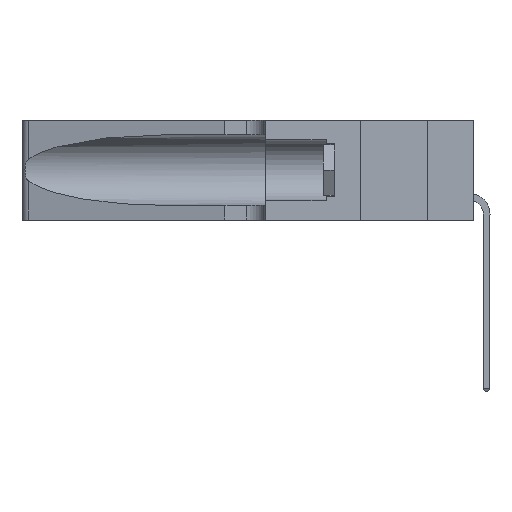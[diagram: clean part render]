
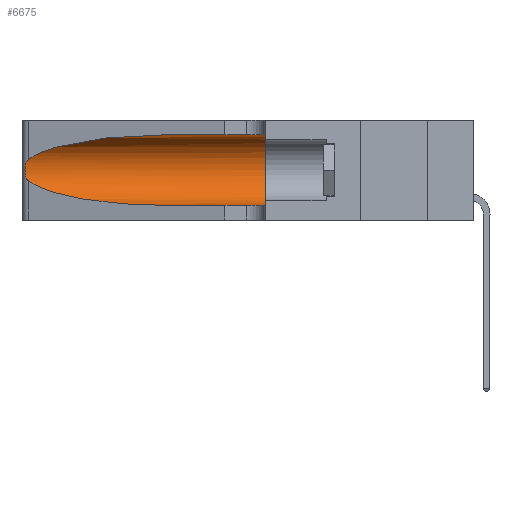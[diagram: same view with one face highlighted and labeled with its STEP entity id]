
A CAD part, left-side view. The second image highlights one B-rep face of the part: STEP entity #6675.
In plain terms, the highlighted cylindrical face has radius 3.308 mm (diameter 6.617 mm), a partial arc.
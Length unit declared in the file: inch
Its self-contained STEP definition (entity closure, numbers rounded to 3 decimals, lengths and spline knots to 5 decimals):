
#290 = LINE ( 'NONE', #19029, #35016 ) ;
#649 = CARTESIAN_POINT ( 'NONE',  ( 0.25639, 1.23186, 0.15144 ) ) ;
#1026 = AXIS2_PLACEMENT_3D ( 'NONE', #22013, #27946, #5043 ) ;
#2391 = ORIENTED_EDGE ( 'NONE', *, *, #7420, .T. ) ;
#3437 = VERTEX_POINT ( 'NONE', #31446 ) ;
#3533 = EDGE_LOOP ( 'NONE', ( #34411, #16324, #2391, #28532, #27664, #22790 ) ) ;
#3738 = CARTESIAN_POINT ( 'NONE',  ( 0.1305, 0.35, 0.185 ) ) ;
#4274 = FACE_OUTER_BOUND ( 'NONE', #3533, .T. ) ;
#4595 = CARTESIAN_POINT ( 'NONE',  ( 0.25487, 1.22718, 0.22369 ) ) ;
#4828 = CARTESIAN_POINT ( 'NONE',  ( 0.1305, 0.72297, 0.05475 ) ) ;
#5043 = DIRECTION ( 'NONE',  ( 0., 0., -1. ) ) ;
#5777 = CARTESIAN_POINT ( 'NONE',  ( 0.25487, 1.22718, 0.14631 ) ) ;
#6529 = CARTESIAN_POINT ( 'NONE',  ( 0.25787, 1.23484, 0.2124 ) ) ;
#6650 = CARTESIAN_POINT ( 'NONE',  ( 0.25487, 1.22718, 0.22369 ) ) ;
#6675 = ADVANCED_FACE ( 'NONE', ( #4274 ), #30547, .F. ) ;
#7420 = EDGE_CURVE ( 'NONE', #35359, #28461, #30790, .T. ) ;
#7726 = LINE ( 'NONE', #19507, #14611 ) ;
#9738 = CARTESIAN_POINT ( 'NONE',  ( 0.26075, 1.23896, 0.178 ) ) ;
#9797 = DIRECTION ( 'NONE',  ( 0., 0., 1. ) ) ;
#9862 = CARTESIAN_POINT ( 'NONE',  ( 0.25487, 1.22718, 0.14631 ) ) ;
#11283 = DIRECTION ( 'NONE',  ( 0., -1., 0. ) ) ;
#11752 = VERTEX_POINT ( 'NONE', #23647 ) ;
#12164 = CARTESIAN_POINT ( 'NONE',  ( 0.2373, 1.15595, 0.28018 ) ) ;
#12416 = CARTESIAN_POINT ( 'NONE',  ( 0.26018, 1.23835, 0.19895 ) ) ;
#12541 = CARTESIAN_POINT ( 'NONE',  ( 0.25854, 1.2359, 0.20912 ) ) ;
#12600 = EDGE_CURVE ( 'NONE', #30801, #11752, #290, .T. ) ;
#12808 = CARTESIAN_POINT ( 'NONE',  ( 0.25555, 1.22993, 0.14849 ) ) ;
#14267 =( BOUNDED_CURVE ( )  B_SPLINE_CURVE ( 3, ( #22950, #29821, #12164, #14772 ),
 .UNSPECIFIED., .F., .F. ) 
 B_SPLINE_CURVE_WITH_KNOTS ( ( 4, 4 ),
 ( 1.5708, 2.84003 ),
 .UNSPECIFIED. ) 
 CURVE ( )  GEOMETRIC_REPRESENTATION_ITEM ( )  RATIONAL_B_SPLINE_CURVE ( ( 1., 0.87, 0.87, 1. ) ) 
 REPRESENTATION_ITEM ( '' )  );
#14611 = VECTOR ( 'NONE', #11283, 39.37008 ) ;
#14772 = CARTESIAN_POINT ( 'NONE',  ( 0.25487, 1.22718, 0.22369 ) ) ;
#15899 = CARTESIAN_POINT ( 'NONE',  ( 0.25856, 1.23593, 0.16098 ) ) ;
#16324 = ORIENTED_EDGE ( 'NONE', *, *, #35091, .T. ) ;
#16944 = CARTESIAN_POINT ( 'NONE',  ( 0.18966, 0.96281, 0.05475 ) ) ;
#17275 = CARTESIAN_POINT ( 'NONE',  ( 0.1305, 0.72297, 0.31525 ) ) ;
#17881 = EDGE_CURVE ( 'NONE', #28461, #3437, #7726, .T. ) ;
#19029 = CARTESIAN_POINT ( 'NONE',  ( 0.1305, 1.61858, 0.31525 ) ) ;
#19507 = CARTESIAN_POINT ( 'NONE',  ( 0.1305, 1.61858, 0.05475 ) ) ;
#20096 = CARTESIAN_POINT ( 'NONE',  ( 0.1305, 0.72297, 0.05475 ) ) ;
#20155 = EDGE_CURVE ( 'NONE', #11752, #3437, #23544, .T. ) ;
#20825 = EDGE_CURVE ( 'NONE', #30801, #23035, #14267, .T. ) ;
#21722 = CARTESIAN_POINT ( 'NONE',  ( 0.26017, 1.23833, 0.17102 ) ) ;
#22013 = CARTESIAN_POINT ( 'NONE',  ( 0.1305, 1.61858, 0.185 ) ) ;
#22790 = ORIENTED_EDGE ( 'NONE', *, *, #12600, .F. ) ;
#22950 = CARTESIAN_POINT ( 'NONE',  ( 0.1305, 0.72297, 0.31525 ) ) ;
#23035 = VERTEX_POINT ( 'NONE', #4595 ) ;
#23544 = CIRCLE ( 'NONE', #31041, 0.13025 ) ;
#23647 = CARTESIAN_POINT ( 'NONE',  ( 0.1305, 0.35, 0.31525 ) ) ;
#24395 = DIRECTION ( 'NONE',  ( 0., 1., 0. ) ) ;
#24717 = CARTESIAN_POINT ( 'NONE',  ( 0.25555, 1.22994, 0.2215 ) ) ;
#27162 = CARTESIAN_POINT ( 'NONE',  ( 0.25639, 1.23184, 0.21858 ) ) ;
#27530 = CARTESIAN_POINT ( 'NONE',  ( 0.26075, 1.23896, 0.19203 ) ) ;
#27664 = ORIENTED_EDGE ( 'NONE', *, *, #20155, .F. ) ;
#27946 = DIRECTION ( 'NONE',  ( 0., -1., 0. ) ) ;
#27949 = DIRECTION ( 'NONE',  ( 0., -1., 0. ) ) ;
#28461 = VERTEX_POINT ( 'NONE', #20096 ) ;
#28532 = ORIENTED_EDGE ( 'NONE', *, *, #17881, .T. ) ;
#29821 = CARTESIAN_POINT ( 'NONE',  ( 0.18966, 0.96281, 0.31525 ) ) ;
#30547 = CYLINDRICAL_SURFACE ( 'NONE', #1026, 0.13025 ) ;
#30790 =( BOUNDED_CURVE ( )  B_SPLINE_CURVE ( 3, ( #37228, #37386, #16944, #4828 ),
 .UNSPECIFIED., .F., .T. ) 
 B_SPLINE_CURVE_WITH_KNOTS ( ( 4, 4 ),
 ( 3.44316, 4.71239 ),
 .UNSPECIFIED. ) 
 CURVE ( )  GEOMETRIC_REPRESENTATION_ITEM ( )  RATIONAL_B_SPLINE_CURVE ( ( 1., 0.87, 0.87, 1. ) ) 
 REPRESENTATION_ITEM ( '' )  );
#30801 = VERTEX_POINT ( 'NONE', #17275 ) ;
#31041 = AXIS2_PLACEMENT_3D ( 'NONE', #3738, #24395, #9797 ) ;
#31446 = CARTESIAN_POINT ( 'NONE',  ( 0.1305, 0.35, 0.05475 ) ) ;
#33192 = CARTESIAN_POINT ( 'NONE',  ( 0.25789, 1.23486, 0.15765 ) ) ;
#33658 = B_SPLINE_CURVE_WITH_KNOTS ( 'NONE', 3,
 ( #6650, #24717, #27162, #6529, #12541, #12416, #27530, #9738, #21722, #15899, #33192, #649, #12808, #9862 ),
 .UNSPECIFIED., .F., .F.,
 ( 4, 2, 2, 2, 2, 2, 4 ),
 ( 0., 0.00027, 0.00053, 0.00107, 0.0016, 0.00187, 0.00214 ),
 .UNSPECIFIED. ) ;
#34411 = ORIENTED_EDGE ( 'NONE', *, *, #20825, .T. ) ;
#35016 = VECTOR ( 'NONE', #27949, 39.37008 ) ;
#35091 = EDGE_CURVE ( 'NONE', #23035, #35359, #33658, .T. ) ;
#35359 = VERTEX_POINT ( 'NONE', #5777 ) ;
#37228 = CARTESIAN_POINT ( 'NONE',  ( 0.25487, 1.22718, 0.14631 ) ) ;
#37386 = CARTESIAN_POINT ( 'NONE',  ( 0.2373, 1.15595, 0.08982 ) ) ;
